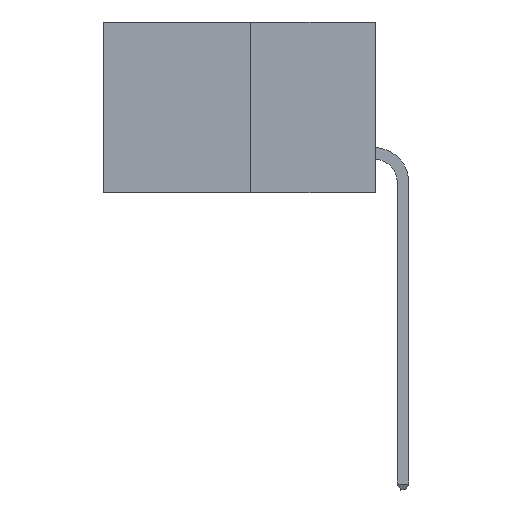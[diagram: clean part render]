
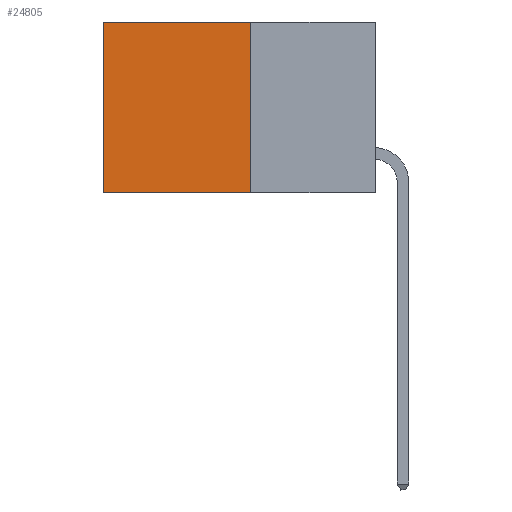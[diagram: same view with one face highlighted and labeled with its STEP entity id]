
A CAD part, left-side view. The second image highlights one B-rep face of the part: STEP entity #24805.
In plain terms, the highlighted planar face has unit normal (-1, 0, 0).
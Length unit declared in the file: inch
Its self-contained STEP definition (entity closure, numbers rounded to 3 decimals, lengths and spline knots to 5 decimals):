
#98 = VECTOR ( 'NONE', #14674, 39.37008 ) ;
#419 = CARTESIAN_POINT ( 'NONE',  ( 0.277, 0.27, -0.37 ) ) ;
#435 = LINE ( 'NONE', #419, #19622 ) ;
#1869 = EDGE_CURVE ( 'NONE', #18394, #26941, #4101, .T. ) ;
#2160 = PLANE ( 'NONE',  #13894 ) ;
#2839 = CARTESIAN_POINT ( 'NONE',  ( 0.277, 0.27, -0.37 ) ) ;
#4101 = LINE ( 'NONE', #15632, #15379 ) ;
#5932 = ORIENTED_EDGE ( 'NONE', *, *, #10388, .T. ) ;
#6702 = CARTESIAN_POINT ( 'NONE',  ( 0.277, 0.27, 0. ) ) ;
#7007 = ORIENTED_EDGE ( 'NONE', *, *, #1869, .F. ) ;
#7020 = CARTESIAN_POINT ( 'NONE',  ( 0.277, 0.27, -0.37 ) ) ;
#8496 = ORIENTED_EDGE ( 'NONE', *, *, #25614, .T. ) ;
#9403 = DIRECTION ( 'NONE',  ( 0., 0., -1. ) ) ;
#9588 = EDGE_LOOP ( 'NONE', ( #8496, #17020, #7007, #5932 ) ) ;
#10388 = EDGE_CURVE ( 'NONE', #18394, #26827, #15194, .T. ) ;
#10636 = CARTESIAN_POINT ( 'NONE',  ( 0.277, 0.59, -0.37 ) ) ;
#10714 = DIRECTION ( 'NONE',  ( 0., 1., 0. ) ) ;
#12855 = LINE ( 'NONE', #28932, #98 ) ;
#12922 = FACE_OUTER_BOUND ( 'NONE', #9588, .T. ) ;
#13894 = AXIS2_PLACEMENT_3D ( 'NONE', #7020, #23795, #9403 ) ;
#14674 = DIRECTION ( 'NONE',  ( 0., 0., -1. ) ) ;
#15194 = LINE ( 'NONE', #23220, #27134 ) ;
#15379 = VECTOR ( 'NONE', #19144, 39.37008 ) ;
#15632 = CARTESIAN_POINT ( 'NONE',  ( 0.277, 0.27, -0.37 ) ) ;
#17020 = ORIENTED_EDGE ( 'NONE', *, *, #26936, .F. ) ;
#18394 = VERTEX_POINT ( 'NONE', #6702 ) ;
#19144 = DIRECTION ( 'NONE',  ( 0., 0., -1. ) ) ;
#19558 = DIRECTION ( 'NONE',  ( 0., 1., 0. ) ) ;
#19622 = VECTOR ( 'NONE', #19558, 39.37008 ) ;
#23220 = CARTESIAN_POINT ( 'NONE',  ( 0.277, 0.27, 0. ) ) ;
#23795 = DIRECTION ( 'NONE',  ( 1., 0., 0. ) ) ;
#23828 = VERTEX_POINT ( 'NONE', #10636 ) ;
#24805 = ADVANCED_FACE ( 'NONE', ( #12922 ), #2160, .F. ) ;
#25614 = EDGE_CURVE ( 'NONE', #26827, #23828, #12855, .T. ) ;
#26306 = CARTESIAN_POINT ( 'NONE',  ( 0.277, 0.59, 0. ) ) ;
#26827 = VERTEX_POINT ( 'NONE', #26306 ) ;
#26936 = EDGE_CURVE ( 'NONE', #26941, #23828, #435, .T. ) ;
#26941 = VERTEX_POINT ( 'NONE', #2839 ) ;
#27134 = VECTOR ( 'NONE', #10714, 39.37008 ) ;
#28932 = CARTESIAN_POINT ( 'NONE',  ( 0.277, 0.59, -0.37 ) ) ;
